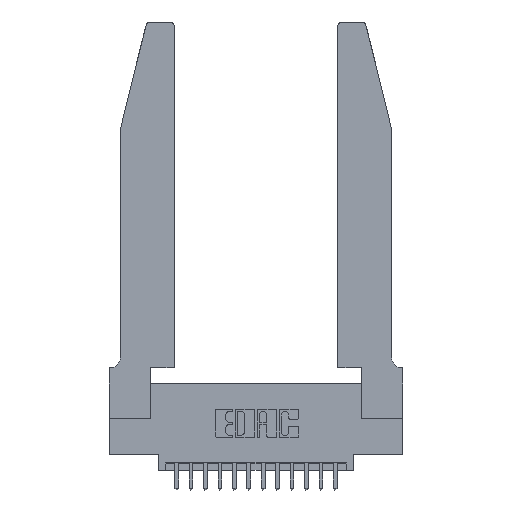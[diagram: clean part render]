
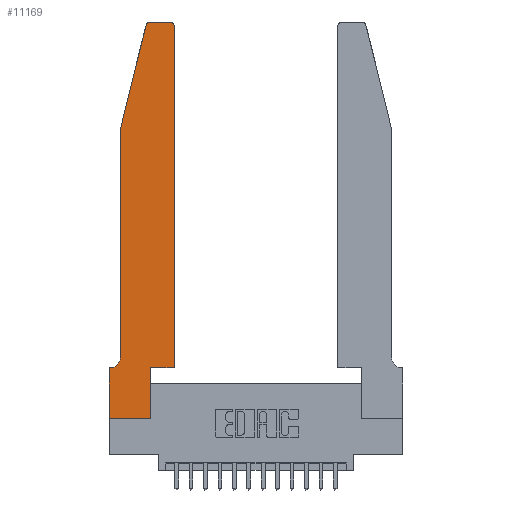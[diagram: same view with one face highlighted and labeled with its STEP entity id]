
A CAD part, top view. The second image highlights one B-rep face of the part: STEP entity #11169.
In plain terms, the highlighted planar face has unit normal (0, 0, 1).
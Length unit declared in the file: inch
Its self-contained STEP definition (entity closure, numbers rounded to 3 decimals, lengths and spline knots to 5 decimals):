
#413 = VERTEX_POINT ( 'NONE', #5623 ) ;
#443 = VERTEX_POINT ( 'NONE', #16939 ) ;
#547 = DIRECTION ( 'NONE',  ( -0.239, -0.971, 0. ) ) ;
#592 = CARTESIAN_POINT ( 'NONE',  ( 0.4505, 2.72, 0.37 ) ) ;
#1012 = DIRECTION ( 'NONE',  ( -1., 0., 0. ) ) ;
#1180 = AXIS2_PLACEMENT_3D ( 'NONE', #2141, #7813, #14845 ) ;
#1213 = ORIENTED_EDGE ( 'NONE', *, *, #5586, .T. ) ;
#1375 = LINE ( 'NONE', #5168, #4294 ) ;
#1414 = DIRECTION ( 'NONE',  ( -1., 0., 0. ) ) ;
#1491 = CARTESIAN_POINT ( 'NONE',  ( 0.2865, 0., 0.37 ) ) ;
#1504 = DIRECTION ( 'NONE',  ( 0., 0., 1. ) ) ;
#1581 = VECTOR ( 'NONE', #10028, 39.37008 ) ;
#1694 = ORIENTED_EDGE ( 'NONE', *, *, #4747, .T. ) ;
#1784 = CARTESIAN_POINT ( 'NONE',  ( 0., 0., 0.37 ) ) ;
#2009 = VECTOR ( 'NONE', #13653, 39.37008 ) ;
#2141 = CARTESIAN_POINT ( 'NONE',  ( 0.4205, 2.72, 0.37 ) ) ;
#2178 = CIRCLE ( 'NONE', #16888, 0.03 ) ;
#2240 = ORIENTED_EDGE ( 'NONE', *, *, #5043, .T. ) ;
#2404 = LINE ( 'NONE', #13022, #9733 ) ;
#2848 = CARTESIAN_POINT ( 'NONE',  ( 0.25487, 2.72718, 0.37 ) ) ;
#3198 = VERTEX_POINT ( 'NONE', #10097 ) ;
#3521 = EDGE_CURVE ( 'NONE', #4672, #11093, #1375, .T. ) ;
#3695 = ORIENTED_EDGE ( 'NONE', *, *, #7339, .T. ) ;
#3868 = DIRECTION ( 'NONE',  ( 0., 1., 0. ) ) ;
#3871 = LINE ( 'NONE', #15825, #1581 ) ;
#4294 = VECTOR ( 'NONE', #3868, 39.37008 ) ;
#4367 = AXIS2_PLACEMENT_3D ( 'NONE', #6706, #16681, #16561 ) ;
#4528 = VERTEX_POINT ( 'NONE', #9653 ) ;
#4672 = VERTEX_POINT ( 'NONE', #1491 ) ;
#4747 = EDGE_CURVE ( 'NONE', #11123, #9827, #11812, .T. ) ;
#5004 = LINE ( 'NONE', #11915, #18053 ) ;
#5034 = CARTESIAN_POINT ( 'NONE',  ( 0.4205, 2.75, 0.37 ) ) ;
#5043 = EDGE_CURVE ( 'NONE', #443, #12154, #7839, .T. ) ;
#5168 = CARTESIAN_POINT ( 'NONE',  ( 0.2865, 0.35, 0.37 ) ) ;
#5261 = EDGE_CURVE ( 'NONE', #15167, #3198, #10935, .T. ) ;
#5586 = EDGE_CURVE ( 'NONE', #413, #15081, #14231, .T. ) ;
#5623 = CARTESIAN_POINT ( 'NONE',  ( 0.4505, 0.35, 0.37 ) ) ;
#5733 = LINE ( 'NONE', #7820, #10385 ) ;
#5951 = DIRECTION ( 'NONE',  ( 0., -1., 0. ) ) ;
#6321 = ORIENTED_EDGE ( 'NONE', *, *, #11010, .T. ) ;
#6706 = CARTESIAN_POINT ( 'NONE',  ( 0.0055, 0.42, 0.37 ) ) ;
#6961 = ORIENTED_EDGE ( 'NONE', *, *, #5261, .T. ) ;
#7039 = EDGE_CURVE ( 'NONE', #15081, #11123, #7985, .T. ) ;
#7053 = PLANE ( 'NONE',  #10160 ) ;
#7339 = EDGE_CURVE ( 'NONE', #9827, #15433, #2178, .T. ) ;
#7813 = DIRECTION ( 'NONE',  ( 0., 0., 1. ) ) ;
#7820 = CARTESIAN_POINT ( 'NONE',  ( 0., 0., 0.37 ) ) ;
#7839 = LINE ( 'NONE', #1784, #9621 ) ;
#7985 = CIRCLE ( 'NONE', #1180, 0.03 ) ;
#8124 = DIRECTION ( 'NONE',  ( 0., 0., 1. ) ) ;
#8248 = ORIENTED_EDGE ( 'NONE', *, *, #17601, .T. ) ;
#8918 = VECTOR ( 'NONE', #1012, 39.37008 ) ;
#9481 = CARTESIAN_POINT ( 'NONE',  ( 0., 0.35, 0.37 ) ) ;
#9545 = CARTESIAN_POINT ( 'NONE',  ( 0.2605, 2.75, 0.37 ) ) ;
#9621 = VECTOR ( 'NONE', #10551, 39.37008 ) ;
#9653 = CARTESIAN_POINT ( 'NONE',  ( 0.0755, 2., 0.37 ) ) ;
#9659 = EDGE_CURVE ( 'NONE', #3198, #443, #15712, .T. ) ;
#9682 = CARTESIAN_POINT ( 'NONE',  ( 0.284, 2.72, 0.37 ) ) ;
#9733 = VECTOR ( 'NONE', #5951, 39.37008 ) ;
#9827 = VERTEX_POINT ( 'NONE', #16005 ) ;
#9954 = FACE_OUTER_BOUND ( 'NONE', #13139, .T. ) ;
#10028 = DIRECTION ( 'NONE',  ( 1., 0., 0. ) ) ;
#10097 = CARTESIAN_POINT ( 'NONE',  ( 0.0055, 0.35, 0.37 ) ) ;
#10160 = AXIS2_PLACEMENT_3D ( 'NONE', #9481, #8124, #12315 ) ;
#10385 = VECTOR ( 'NONE', #12012, 39.37008 ) ;
#10531 = CARTESIAN_POINT ( 'NONE',  ( 0.2865, 0.35, 0.37 ) ) ;
#10551 = DIRECTION ( 'NONE',  ( 0., -1., 0. ) ) ;
#10683 = ORIENTED_EDGE ( 'NONE', *, *, #9659, .T. ) ;
#10719 = ORIENTED_EDGE ( 'NONE', *, *, #7039, .T. ) ;
#10935 = CIRCLE ( 'NONE', #4367, 0.07 ) ;
#11010 = EDGE_CURVE ( 'NONE', #12154, #4672, #5733, .T. ) ;
#11093 = VERTEX_POINT ( 'NONE', #10531 ) ;
#11123 = VERTEX_POINT ( 'NONE', #5034 ) ;
#11169 = ADVANCED_FACE ( 'NONE', ( #9954 ), #7053, .T. ) ;
#11274 = DIRECTION ( 'NONE',  ( 1., 0., 0. ) ) ;
#11812 = LINE ( 'NONE', #9545, #8918 ) ;
#11915 = CARTESIAN_POINT ( 'NONE',  ( 0.0755, 2., 0.37 ) ) ;
#12012 = DIRECTION ( 'NONE',  ( 1., 0., 0. ) ) ;
#12034 = EDGE_CURVE ( 'NONE', #4528, #15167, #2404, .T. ) ;
#12042 = ORIENTED_EDGE ( 'NONE', *, *, #12034, .T. ) ;
#12154 = VERTEX_POINT ( 'NONE', #16121 ) ;
#12315 = DIRECTION ( 'NONE',  ( 1., 0., 0. ) ) ;
#13022 = CARTESIAN_POINT ( 'NONE',  ( 0.0755, 2., 0.37 ) ) ;
#13139 = EDGE_LOOP ( 'NONE', ( #1694, #3695, #16018, #12042, #6961, #10683, #2240, #6321, #16868, #8248, #1213, #10719 ) ) ;
#13590 = CARTESIAN_POINT ( 'NONE',  ( 0.4505, 0.35, 0.37 ) ) ;
#13653 = DIRECTION ( 'NONE',  ( 0., 1., 0. ) ) ;
#14231 = LINE ( 'NONE', #13590, #2009 ) ;
#14845 = DIRECTION ( 'NONE',  ( 1., 0., 0. ) ) ;
#15081 = VERTEX_POINT ( 'NONE', #592 ) ;
#15167 = VERTEX_POINT ( 'NONE', #17897 ) ;
#15433 = VERTEX_POINT ( 'NONE', #2848 ) ;
#15456 = CARTESIAN_POINT ( 'NONE',  ( 0.0755, 0.35, 0.37 ) ) ;
#15712 = LINE ( 'NONE', #15456, #17047 ) ;
#15825 = CARTESIAN_POINT ( 'NONE',  ( 0.4505, 0.35, 0.37 ) ) ;
#16005 = CARTESIAN_POINT ( 'NONE',  ( 0.284, 2.75, 0.37 ) ) ;
#16018 = ORIENTED_EDGE ( 'NONE', *, *, #16606, .T. ) ;
#16121 = CARTESIAN_POINT ( 'NONE',  ( 0., 0., 0.37 ) ) ;
#16561 = DIRECTION ( 'NONE',  ( -1., 0., 0. ) ) ;
#16606 = EDGE_CURVE ( 'NONE', #15433, #4528, #5004, .T. ) ;
#16681 = DIRECTION ( 'NONE',  ( 0., 0., -1. ) ) ;
#16868 = ORIENTED_EDGE ( 'NONE', *, *, #3521, .T. ) ;
#16888 = AXIS2_PLACEMENT_3D ( 'NONE', #9682, #1504, #11274 ) ;
#16939 = CARTESIAN_POINT ( 'NONE',  ( 0., 0.35, 0.37 ) ) ;
#17047 = VECTOR ( 'NONE', #1414, 39.37008 ) ;
#17601 = EDGE_CURVE ( 'NONE', #11093, #413, #3871, .T. ) ;
#17897 = CARTESIAN_POINT ( 'NONE',  ( 0.0755, 0.42, 0.37 ) ) ;
#18053 = VECTOR ( 'NONE', #547, 39.37008 ) ;
